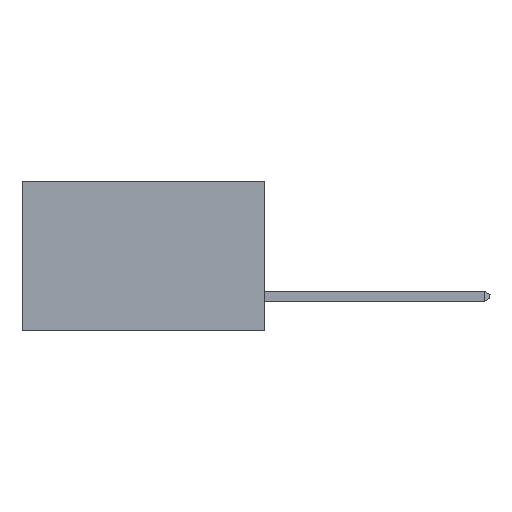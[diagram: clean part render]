
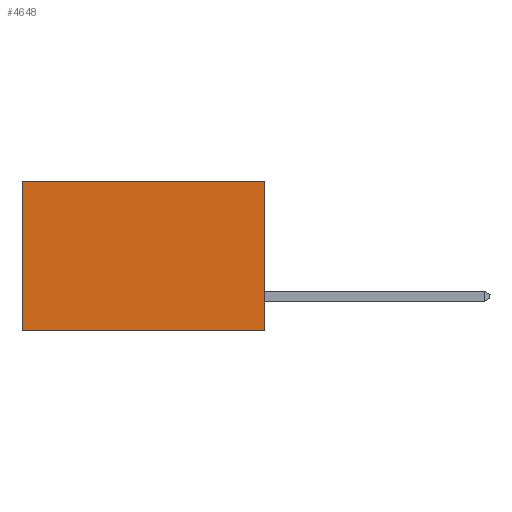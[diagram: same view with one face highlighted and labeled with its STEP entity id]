
A CAD part, left-side view. The second image highlights one B-rep face of the part: STEP entity #4648.
In plain terms, the highlighted planar face has unit normal (-1, 0, 0).
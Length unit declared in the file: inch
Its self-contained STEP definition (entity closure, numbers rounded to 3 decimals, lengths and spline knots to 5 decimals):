
#397 = EDGE_CURVE ( 'NONE', #926, #4155, #5489, .T. ) ;
#576 = DIRECTION ( 'NONE',  ( 0., 0., -1. ) ) ;
#926 = VERTEX_POINT ( 'NONE', #999 ) ;
#964 = ORIENTED_EDGE ( 'NONE', *, *, #4295, .F. ) ;
#999 = CARTESIAN_POINT ( 'NONE',  ( 0.2615, 0., -0.37 ) ) ;
#1087 = CARTESIAN_POINT ( 'NONE',  ( 0.2615, 0.6, -0.37 ) ) ;
#1349 = DIRECTION ( 'NONE',  ( 0., 0., -1. ) ) ;
#2628 = VERTEX_POINT ( 'NONE', #11113 ) ;
#2873 = EDGE_LOOP ( 'NONE', ( #4239, #5677, #964, #5570 ) ) ;
#3001 = VERTEX_POINT ( 'NONE', #5239 ) ;
#3227 = CARTESIAN_POINT ( 'NONE',  ( 0.2615, 0., 0. ) ) ;
#3343 = FACE_OUTER_BOUND ( 'NONE', #2873, .T. ) ;
#4155 = VERTEX_POINT ( 'NONE', #8011 ) ;
#4220 = LINE ( 'NONE', #3227, #7989 ) ;
#4239 = ORIENTED_EDGE ( 'NONE', *, *, #5813, .T. ) ;
#4277 = PLANE ( 'NONE',  #4620 ) ;
#4295 = EDGE_CURVE ( 'NONE', #2628, #926, #5312, .T. ) ;
#4620 = AXIS2_PLACEMENT_3D ( 'NONE', #9132, #10195, #576 ) ;
#4648 = ADVANCED_FACE ( 'NONE', ( #3343 ), #4277, .F. ) ;
#5014 = VECTOR ( 'NONE', #11831, 39.37008 ) ;
#5239 = CARTESIAN_POINT ( 'NONE',  ( 0.2615, 0.6, 0. ) ) ;
#5312 = LINE ( 'NONE', #6198, #10914 ) ;
#5489 = LINE ( 'NONE', #7376, #10704 ) ;
#5570 = ORIENTED_EDGE ( 'NONE', *, *, #6717, .T. ) ;
#5677 = ORIENTED_EDGE ( 'NONE', *, *, #397, .F. ) ;
#5813 = EDGE_CURVE ( 'NONE', #3001, #4155, #7810, .T. ) ;
#6198 = CARTESIAN_POINT ( 'NONE',  ( 0.2615, 0., -0.37 ) ) ;
#6717 = EDGE_CURVE ( 'NONE', #2628, #3001, #4220, .T. ) ;
#7077 = DIRECTION ( 'NONE',  ( 0., 1., 0. ) ) ;
#7376 = CARTESIAN_POINT ( 'NONE',  ( 0.2615, 0., -0.37 ) ) ;
#7810 = LINE ( 'NONE', #1087, #5014 ) ;
#7989 = VECTOR ( 'NONE', #7077, 39.37008 ) ;
#8011 = CARTESIAN_POINT ( 'NONE',  ( 0.2615, 0.6, -0.37 ) ) ;
#9132 = CARTESIAN_POINT ( 'NONE',  ( 0.2615, 0., -0.37 ) ) ;
#10195 = DIRECTION ( 'NONE',  ( 1., 0., 0. ) ) ;
#10704 = VECTOR ( 'NONE', #12274, 39.37008 ) ;
#10914 = VECTOR ( 'NONE', #1349, 39.37008 ) ;
#11113 = CARTESIAN_POINT ( 'NONE',  ( 0.2615, 0., 0. ) ) ;
#11831 = DIRECTION ( 'NONE',  ( 0., 0., -1. ) ) ;
#12274 = DIRECTION ( 'NONE',  ( 0., 1., 0. ) ) ;
